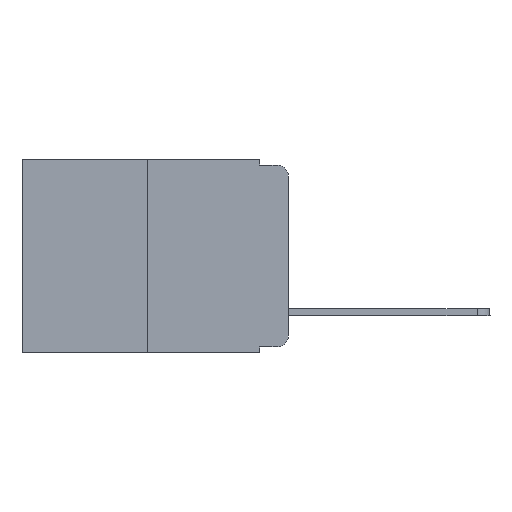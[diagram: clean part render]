
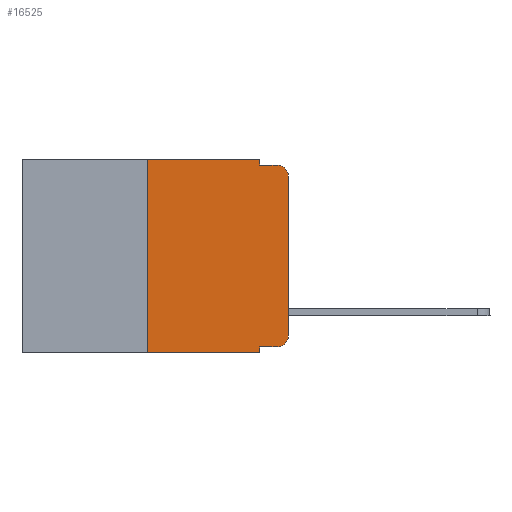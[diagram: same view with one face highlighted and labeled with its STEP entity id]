
A CAD part, left-side view. The second image highlights one B-rep face of the part: STEP entity #16525.
In plain terms, the highlighted planar face has unit normal (-1, 0, 0).
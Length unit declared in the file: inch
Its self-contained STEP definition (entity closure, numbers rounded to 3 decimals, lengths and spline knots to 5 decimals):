
#41 = DIRECTION ( 'NONE',  ( 0., 0., 1. ) ) ;
#178 = ORIENTED_EDGE ( 'NONE', *, *, #8744, .T. ) ;
#750 = CARTESIAN_POINT ( 'NONE',  ( 0., 0.02, -0.333 ) ) ;
#759 = EDGE_CURVE ( 'NONE', #1960, #16394, #9866, .T. ) ;
#762 = EDGE_CURVE ( 'NONE', #16057, #7276, #13168, .T. ) ;
#1326 = AXIS2_PLACEMENT_3D ( 'NONE', #4630, #15600, #5948 ) ;
#1363 = PLANE ( 'NONE',  #9240 ) ;
#1475 = DIRECTION ( 'NONE',  ( 0., 0., -1. ) ) ;
#1540 = ORIENTED_EDGE ( 'NONE', *, *, #762, .T. ) ;
#1906 = VECTOR ( 'NONE', #18010, 39.37008 ) ;
#1960 = VERTEX_POINT ( 'NONE', #9155 ) ;
#2380 = CARTESIAN_POINT ( 'NONE',  ( 0., 0., -0.03 ) ) ;
#2602 = VECTOR ( 'NONE', #7305, 39.37008 ) ;
#2920 = VECTOR ( 'NONE', #7445, 39.37008 ) ;
#3498 = ORIENTED_EDGE ( 'NONE', *, *, #16228, .T. ) ;
#3693 = VERTEX_POINT ( 'NONE', #2380 ) ;
#4527 = DIRECTION ( 'NONE',  ( 0., 0., -1. ) ) ;
#4630 = CARTESIAN_POINT ( 'NONE',  ( 0., 0.02, -0.03 ) ) ;
#5232 = ORIENTED_EDGE ( 'NONE', *, *, #759, .F. ) ;
#5948 = DIRECTION ( 'NONE',  ( 0., 0., -1. ) ) ;
#6284 = LINE ( 'NONE', #8434, #14335 ) ;
#6468 = LINE ( 'NONE', #16616, #1906 ) ;
#6542 = ORIENTED_EDGE ( 'NONE', *, *, #6796, .T. ) ;
#6549 = CARTESIAN_POINT ( 'NONE',  ( 0., 0., 0. ) ) ;
#6714 = LINE ( 'NONE', #15692, #2602 ) ;
#6796 = EDGE_CURVE ( 'NONE', #3693, #16394, #16785, .T. ) ;
#6962 = CARTESIAN_POINT ( 'NONE',  ( 0., 0.051, -0.343 ) ) ;
#7093 = CARTESIAN_POINT ( 'NONE',  ( 0., 0.02, -0.01 ) ) ;
#7276 = VERTEX_POINT ( 'NONE', #7878 ) ;
#7305 = DIRECTION ( 'NONE',  ( 0., -1., 0. ) ) ;
#7356 = CARTESIAN_POINT ( 'NONE',  ( 0., 0.051, 0. ) ) ;
#7445 = DIRECTION ( 'NONE',  ( 0., -1., 0. ) ) ;
#7865 = LINE ( 'NONE', #9518, #17480 ) ;
#7878 = CARTESIAN_POINT ( 'NONE',  ( 0., 0., -0.313 ) ) ;
#8177 = LINE ( 'NONE', #17246, #15201 ) ;
#8304 = EDGE_LOOP ( 'NONE', ( #16149, #6542, #5232, #17948, #11413, #14486, #178, #12132, #3498, #1540 ) ) ;
#8399 = VECTOR ( 'NONE', #9125, 39.37008 ) ;
#8434 = CARTESIAN_POINT ( 'NONE',  ( 0., 0.051, 0. ) ) ;
#8448 = CARTESIAN_POINT ( 'NONE',  ( 0., 0.25, -0.343 ) ) ;
#8612 = LINE ( 'NONE', #16043, #8399 ) ;
#8744 = EDGE_CURVE ( 'NONE', #16206, #11958, #8612, .T. ) ;
#9125 = DIRECTION ( 'NONE',  ( 0., -1., 0. ) ) ;
#9155 = CARTESIAN_POINT ( 'NONE',  ( 0., 0.051, -0.01 ) ) ;
#9240 = AXIS2_PLACEMENT_3D ( 'NONE', #11155, #9923, #1475 ) ;
#9518 = CARTESIAN_POINT ( 'NONE',  ( 0., 0.25, 0. ) ) ;
#9866 = LINE ( 'NONE', #10316, #2920 ) ;
#9923 = DIRECTION ( 'NONE',  ( 1., 0., 0. ) ) ;
#10316 = CARTESIAN_POINT ( 'NONE',  ( 0., 0.051, -0.01 ) ) ;
#10977 = DIRECTION ( 'NONE',  ( 0., 0., 1. ) ) ;
#10981 = EDGE_CURVE ( 'NONE', #7276, #3693, #12509, .T. ) ;
#11155 = CARTESIAN_POINT ( 'NONE',  ( 0., 0.473, 0. ) ) ;
#11413 = ORIENTED_EDGE ( 'NONE', *, *, #17707, .F. ) ;
#11731 = CARTESIAN_POINT ( 'NONE',  ( 0., 0.25, 0. ) ) ;
#11958 = VERTEX_POINT ( 'NONE', #6962 ) ;
#12132 = ORIENTED_EDGE ( 'NONE', *, *, #16347, .F. ) ;
#12509 = LINE ( 'NONE', #6549, #14955 ) ;
#13168 = CIRCLE ( 'NONE', #17950, 0.02 ) ;
#13935 = CARTESIAN_POINT ( 'NONE',  ( 0., 0.02, -0.313 ) ) ;
#13993 = DIRECTION ( 'NONE',  ( 0., 0., -1. ) ) ;
#14247 = DIRECTION ( 'NONE',  ( -1., 0., 0. ) ) ;
#14251 = CARTESIAN_POINT ( 'NONE',  ( 0., 0.051, -0.333 ) ) ;
#14335 = VECTOR ( 'NONE', #16703, 39.37008 ) ;
#14486 = ORIENTED_EDGE ( 'NONE', *, *, #14705, .F. ) ;
#14705 = EDGE_CURVE ( 'NONE', #16206, #18038, #7865, .T. ) ;
#14955 = VECTOR ( 'NONE', #41, 39.37008 ) ;
#15201 = VECTOR ( 'NONE', #4527, 39.37008 ) ;
#15231 = FACE_OUTER_BOUND ( 'NONE', #8304, .T. ) ;
#15522 = VERTEX_POINT ( 'NONE', #7356 ) ;
#15600 = DIRECTION ( 'NONE',  ( -1., 0., 0. ) ) ;
#15692 = CARTESIAN_POINT ( 'NONE',  ( 0., 0.051, -0.333 ) ) ;
#16043 = CARTESIAN_POINT ( 'NONE',  ( 0., 0.473, -0.343 ) ) ;
#16057 = VERTEX_POINT ( 'NONE', #750 ) ;
#16149 = ORIENTED_EDGE ( 'NONE', *, *, #10981, .T. ) ;
#16206 = VERTEX_POINT ( 'NONE', #8448 ) ;
#16228 = EDGE_CURVE ( 'NONE', #17303, #16057, #6714, .T. ) ;
#16347 = EDGE_CURVE ( 'NONE', #17303, #11958, #6284, .T. ) ;
#16394 = VERTEX_POINT ( 'NONE', #7093 ) ;
#16525 = ADVANCED_FACE ( 'NONE', ( #15231 ), #1363, .F. ) ;
#16616 = CARTESIAN_POINT ( 'NONE',  ( 0., 0.473, 0. ) ) ;
#16703 = DIRECTION ( 'NONE',  ( 0., 0., -1. ) ) ;
#16785 = CIRCLE ( 'NONE', #1326, 0.02 ) ;
#17246 = CARTESIAN_POINT ( 'NONE',  ( 0., 0.051, 0. ) ) ;
#17303 = VERTEX_POINT ( 'NONE', #14251 ) ;
#17355 = EDGE_CURVE ( 'NONE', #15522, #1960, #8177, .T. ) ;
#17480 = VECTOR ( 'NONE', #10977, 39.37008 ) ;
#17707 = EDGE_CURVE ( 'NONE', #18038, #15522, #6468, .T. ) ;
#17948 = ORIENTED_EDGE ( 'NONE', *, *, #17355, .F. ) ;
#17950 = AXIS2_PLACEMENT_3D ( 'NONE', #13935, #14247, #13993 ) ;
#18010 = DIRECTION ( 'NONE',  ( 0., -1., 0. ) ) ;
#18038 = VERTEX_POINT ( 'NONE', #11731 ) ;
